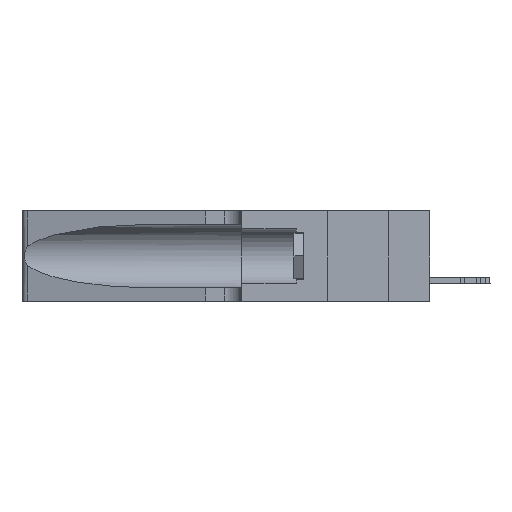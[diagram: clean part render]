
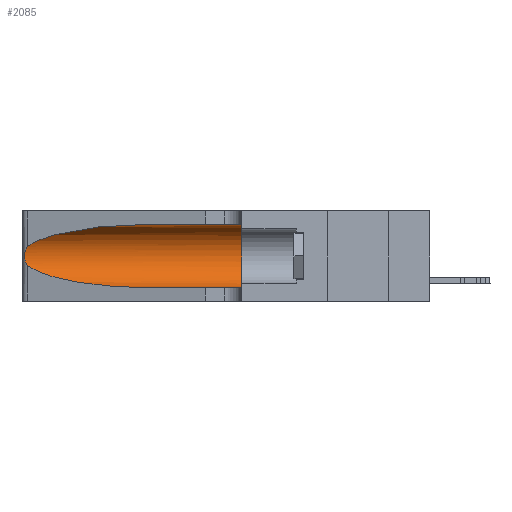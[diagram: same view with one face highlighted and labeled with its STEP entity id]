
A CAD part, left-side view. The second image highlights one B-rep face of the part: STEP entity #2085.
In plain terms, the highlighted cylindrical face has radius 3.308 mm (diameter 6.617 mm), a partial arc.
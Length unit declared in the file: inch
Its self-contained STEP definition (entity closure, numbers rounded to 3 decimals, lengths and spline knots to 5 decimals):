
#2085 = ADVANCED_FACE ( 'NONE', ( #15388 ), #27252, .F. ) ;
#2634 = VERTEX_POINT ( 'NONE', #2660 ) ;
#2660 = CARTESIAN_POINT ( 'NONE',  ( 0.1305, 0.35, 0.05475 ) ) ;
#2767 = CIRCLE ( 'NONE', #41793, 0.13025 ) ;
#4248 = CARTESIAN_POINT ( 'NONE',  ( 0.25787, 1.23484, 0.2124 ) ) ;
#4256 = VERTEX_POINT ( 'NONE', #28415 ) ;
#6854 = ORIENTED_EDGE ( 'NONE', *, *, #37517, .F. ) ;
#7080 = CARTESIAN_POINT ( 'NONE',  ( 0.2373, 1.15595, 0.08982 ) ) ;
#8894 = ORIENTED_EDGE ( 'NONE', *, *, #20156, .F. ) ;
#8931 = EDGE_CURVE ( 'NONE', #26628, #35591, #45120, .T. ) ;
#9443 = CARTESIAN_POINT ( 'NONE',  ( 0.1305, 1.61858, 0.31525 ) ) ;
#10025 = CARTESIAN_POINT ( 'NONE',  ( 0.1305, 1.61858, 0.05475 ) ) ;
#10947 = DIRECTION ( 'NONE',  ( 0., -1., 0. ) ) ;
#11913 = CARTESIAN_POINT ( 'NONE',  ( 0.26075, 1.23896, 0.19203 ) ) ;
#12074 = CARTESIAN_POINT ( 'NONE',  ( 0.26075, 1.23896, 0.178 ) ) ;
#13673 = CARTESIAN_POINT ( 'NONE',  ( 0.1305, 0.72297, 0.05475 ) ) ;
#15204 = ORIENTED_EDGE ( 'NONE', *, *, #47866, .T. ) ;
#15388 = FACE_OUTER_BOUND ( 'NONE', #41805, .T. ) ;
#16933 = ORIENTED_EDGE ( 'NONE', *, *, #48702, .T. ) ;
#17821 = CARTESIAN_POINT ( 'NONE',  ( 0.1305, 0.72297, 0.05475 ) ) ;
#17887 = CARTESIAN_POINT ( 'NONE',  ( 0.25487, 1.22718, 0.22369 ) ) ;
#18323 = CARTESIAN_POINT ( 'NONE',  ( 0.18966, 0.96281, 0.05475 ) ) ;
#18381 = CARTESIAN_POINT ( 'NONE',  ( 0.2373, 1.15595, 0.28018 ) ) ;
#18521 = B_SPLINE_CURVE_WITH_KNOTS ( 'NONE', 3,
 ( #38381, #34967, #23587, #4248, #34350, #34668, #11913, #12074, #38536, #42055, #46173, #42359, #27287, #19462 ),
 .UNSPECIFIED., .F., .F.,
 ( 4, 2, 2, 2, 2, 2, 4 ),
 ( 0., 0.00027, 0.00053, 0.00107, 0.0016, 0.00187, 0.00214 ),
 .UNSPECIFIED. ) ;
#19462 = CARTESIAN_POINT ( 'NONE',  ( 0.25487, 1.22718, 0.14631 ) ) ;
#20156 = EDGE_CURVE ( 'NONE', #4256, #21857, #34677, .T. ) ;
#20402 = ORIENTED_EDGE ( 'NONE', *, *, #8931, .T. ) ;
#21693 = VECTOR ( 'NONE', #43947, 39.37008 ) ;
#21857 = VERTEX_POINT ( 'NONE', #41700 ) ;
#21882 = DIRECTION ( 'NONE',  ( 0., 1., 0. ) ) ;
#23587 = CARTESIAN_POINT ( 'NONE',  ( 0.25639, 1.23184, 0.21858 ) ) ;
#24093 = CARTESIAN_POINT ( 'NONE',  ( 0.1305, 1.61858, 0.185 ) ) ;
#25195 =( BOUNDED_CURVE ( )  B_SPLINE_CURVE ( 3, ( #32333, #47716, #18381, #17887 ),
 .UNSPECIFIED., .F., .T. ) 
 B_SPLINE_CURVE_WITH_KNOTS ( ( 4, 4 ),
 ( 1.5708, 2.84003 ),
 .UNSPECIFIED. ) 
 CURVE ( )  GEOMETRIC_REPRESENTATION_ITEM ( )  RATIONAL_B_SPLINE_CURVE ( ( 1., 0.87, 0.87, 1. ) ) 
 REPRESENTATION_ITEM ( '' )  );
#25280 = VERTEX_POINT ( 'NONE', #28905 ) ;
#26628 = VERTEX_POINT ( 'NONE', #35399 ) ;
#27252 = CYLINDRICAL_SURFACE ( 'NONE', #48940, 0.13025 ) ;
#27287 = CARTESIAN_POINT ( 'NONE',  ( 0.25555, 1.22993, 0.14849 ) ) ;
#28415 = CARTESIAN_POINT ( 'NONE',  ( 0.1305, 0.72297, 0.31525 ) ) ;
#28905 = CARTESIAN_POINT ( 'NONE',  ( 0.25487, 1.22718, 0.22369 ) ) ;
#29611 = CARTESIAN_POINT ( 'NONE',  ( 0.25487, 1.22718, 0.14631 ) ) ;
#32333 = CARTESIAN_POINT ( 'NONE',  ( 0.1305, 0.72297, 0.31525 ) ) ;
#33164 = DIRECTION ( 'NONE',  ( 0., -1., 0. ) ) ;
#34350 = CARTESIAN_POINT ( 'NONE',  ( 0.25854, 1.2359, 0.20912 ) ) ;
#34668 = CARTESIAN_POINT ( 'NONE',  ( 0.26018, 1.23835, 0.19895 ) ) ;
#34677 = LINE ( 'NONE', #9443, #40068 ) ;
#34967 = CARTESIAN_POINT ( 'NONE',  ( 0.25555, 1.22994, 0.2215 ) ) ;
#35399 = CARTESIAN_POINT ( 'NONE',  ( 0.25487, 1.22718, 0.14631 ) ) ;
#35591 = VERTEX_POINT ( 'NONE', #13673 ) ;
#37300 = CARTESIAN_POINT ( 'NONE',  ( 0.1305, 0.35, 0.185 ) ) ;
#37473 = ORIENTED_EDGE ( 'NONE', *, *, #42161, .T. ) ;
#37517 = EDGE_CURVE ( 'NONE', #21857, #2634, #2767, .T. ) ;
#38381 = CARTESIAN_POINT ( 'NONE',  ( 0.25487, 1.22718, 0.22369 ) ) ;
#38536 = CARTESIAN_POINT ( 'NONE',  ( 0.26017, 1.23833, 0.17102 ) ) ;
#38954 = LINE ( 'NONE', #10025, #21693 ) ;
#40068 = VECTOR ( 'NONE', #33164, 39.37008 ) ;
#41700 = CARTESIAN_POINT ( 'NONE',  ( 0.1305, 0.35, 0.31525 ) ) ;
#41793 = AXIS2_PLACEMENT_3D ( 'NONE', #37300, #21882, #48933 ) ;
#41805 = EDGE_LOOP ( 'NONE', ( #16933, #37473, #20402, #15204, #6854, #8894 ) ) ;
#42055 = CARTESIAN_POINT ( 'NONE',  ( 0.25856, 1.23593, 0.16098 ) ) ;
#42161 = EDGE_CURVE ( 'NONE', #25280, #26628, #18521, .T. ) ;
#42359 = CARTESIAN_POINT ( 'NONE',  ( 0.25639, 1.23186, 0.15144 ) ) ;
#43947 = DIRECTION ( 'NONE',  ( 0., -1., 0. ) ) ;
#43979 = DIRECTION ( 'NONE',  ( 0., 0., -1. ) ) ;
#45120 =( BOUNDED_CURVE ( )  B_SPLINE_CURVE ( 3, ( #29611, #7080, #18323, #17821 ),
 .UNSPECIFIED., .F., .F. ) 
 B_SPLINE_CURVE_WITH_KNOTS ( ( 4, 4 ),
 ( 3.44316, 4.71239 ),
 .UNSPECIFIED. ) 
 CURVE ( )  GEOMETRIC_REPRESENTATION_ITEM ( )  RATIONAL_B_SPLINE_CURVE ( ( 1., 0.87, 0.87, 1. ) ) 
 REPRESENTATION_ITEM ( '' )  );
#46173 = CARTESIAN_POINT ( 'NONE',  ( 0.25789, 1.23486, 0.15765 ) ) ;
#47716 = CARTESIAN_POINT ( 'NONE',  ( 0.18966, 0.96281, 0.31525 ) ) ;
#47866 = EDGE_CURVE ( 'NONE', #35591, #2634, #38954, .T. ) ;
#48702 = EDGE_CURVE ( 'NONE', #4256, #25280, #25195, .T. ) ;
#48933 = DIRECTION ( 'NONE',  ( 0., 0., 1. ) ) ;
#48940 = AXIS2_PLACEMENT_3D ( 'NONE', #24093, #10947, #43979 ) ;
